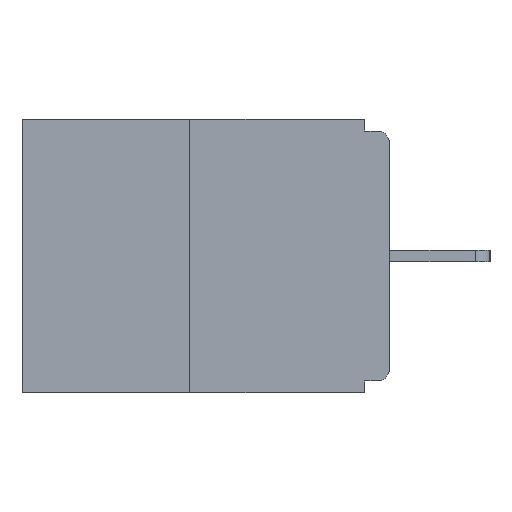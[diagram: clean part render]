
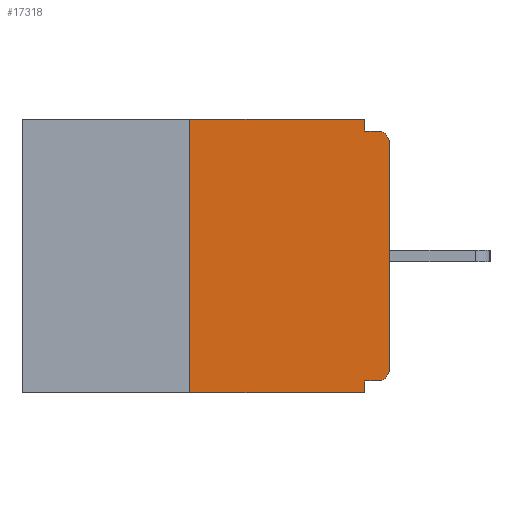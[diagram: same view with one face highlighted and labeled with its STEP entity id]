
A CAD part, left-side view. The second image highlights one B-rep face of the part: STEP entity #17318.
In plain terms, the highlighted planar face has unit normal (-1, 0, 0).
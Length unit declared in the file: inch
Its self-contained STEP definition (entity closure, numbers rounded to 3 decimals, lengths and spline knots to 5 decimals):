
#154 = DIRECTION ( 'NONE',  ( 0., -1., 0. ) ) ;
#231 = DIRECTION ( 'NONE',  ( 0., -1., 0. ) ) ;
#353 = DIRECTION ( 'NONE',  ( 0., 1., 0. ) ) ;
#889 = CARTESIAN_POINT ( 'NONE',  ( 0., 0.031, 0. ) ) ;
#992 = DIRECTION ( 'NONE',  ( 0., 0., -1. ) ) ;
#1017 = VECTOR ( 'NONE', #8878, 39.37008 ) ;
#1216 = VERTEX_POINT ( 'NONE', #3396 ) ;
#1572 = FACE_OUTER_BOUND ( 'NONE', #5780, .T. ) ;
#2127 = VERTEX_POINT ( 'NONE', #9946 ) ;
#2263 = AXIS2_PLACEMENT_3D ( 'NONE', #9028, #4703, #18365 ) ;
#2446 = VERTEX_POINT ( 'NONE', #13920 ) ;
#2466 = CARTESIAN_POINT ( 'NONE',  ( 0., 0.25, 0. ) ) ;
#2790 = LINE ( 'NONE', #10795, #16393 ) ;
#2808 = VECTOR ( 'NONE', #231, 39.37008 ) ;
#3085 = LINE ( 'NONE', #9279, #2808 ) ;
#3396 = CARTESIAN_POINT ( 'NONE',  ( 0., 0.031, -0.343 ) ) ;
#3453 = ORIENTED_EDGE ( 'NONE', *, *, #7222, .F. ) ;
#4030 = EDGE_CURVE ( 'NONE', #13997, #1216, #3085, .T. ) ;
#4128 = ORIENTED_EDGE ( 'NONE', *, *, #18078, .T. ) ;
#4703 = DIRECTION ( 'NONE',  ( -1., 0., 0. ) ) ;
#4943 = CARTESIAN_POINT ( 'NONE',  ( 0., 0., -0.03 ) ) ;
#4972 = LINE ( 'NONE', #18648, #16257 ) ;
#5267 = AXIS2_PLACEMENT_3D ( 'NONE', #12679, #8054, #12485 ) ;
#5558 = VERTEX_POINT ( 'NONE', #19619 ) ;
#5698 = VERTEX_POINT ( 'NONE', #2466 ) ;
#5731 = DIRECTION ( 'NONE',  ( -1., 0., 0. ) ) ;
#5780 = EDGE_LOOP ( 'NONE', ( #3453, #14515, #17949, #17468, #13787, #6718, #7789, #4128, #11120, #6694 ) ) ;
#5939 = DIRECTION ( 'NONE',  ( 0., 0., 1. ) ) ;
#6694 = ORIENTED_EDGE ( 'NONE', *, *, #19433, .F. ) ;
#6718 = ORIENTED_EDGE ( 'NONE', *, *, #12239, .T. ) ;
#6773 = EDGE_CURVE ( 'NONE', #8079, #2127, #4972, .T. ) ;
#6916 = VECTOR ( 'NONE', #17619, 39.37008 ) ;
#6953 = LINE ( 'NONE', #8866, #16837 ) ;
#7222 = EDGE_CURVE ( 'NONE', #5698, #5558, #14438, .T. ) ;
#7484 = VERTEX_POINT ( 'NONE', #16487 ) ;
#7655 = PLANE ( 'NONE',  #5267 ) ;
#7789 = ORIENTED_EDGE ( 'NONE', *, *, #8842, .T. ) ;
#8054 = DIRECTION ( 'NONE',  ( 1., 0., 0. ) ) ;
#8079 = VERTEX_POINT ( 'NONE', #19260 ) ;
#8117 = LINE ( 'NONE', #17078, #18881 ) ;
#8842 = EDGE_CURVE ( 'NONE', #7484, #14604, #8117, .T. ) ;
#8866 = CARTESIAN_POINT ( 'NONE',  ( 0., 0.25, 0. ) ) ;
#8878 = DIRECTION ( 'NONE',  ( 0., 0., -1. ) ) ;
#9028 = CARTESIAN_POINT ( 'NONE',  ( 0., 0.015, -0.313 ) ) ;
#9279 = CARTESIAN_POINT ( 'NONE',  ( 0., 0.46, -0.343 ) ) ;
#9760 = VECTOR ( 'NONE', #992, 39.37008 ) ;
#9946 = CARTESIAN_POINT ( 'NONE',  ( 0., 0.031, -0.328 ) ) ;
#10795 = CARTESIAN_POINT ( 'NONE',  ( 0., 0., -0.015 ) ) ;
#10898 = CARTESIAN_POINT ( 'NONE',  ( 0., 0.25, -0.343 ) ) ;
#11120 = ORIENTED_EDGE ( 'NONE', *, *, #12690, .F. ) ;
#11532 = LINE ( 'NONE', #889, #9760 ) ;
#11969 = CARTESIAN_POINT ( 'NONE',  ( 0., 0.015, -0.03 ) ) ;
#12239 = EDGE_CURVE ( 'NONE', #8079, #7484, #16699, .T. ) ;
#12485 = DIRECTION ( 'NONE',  ( 0., 0., -1. ) ) ;
#12679 = CARTESIAN_POINT ( 'NONE',  ( 0., 0.46, 0. ) ) ;
#12690 = EDGE_CURVE ( 'NONE', #14749, #2446, #2790, .T. ) ;
#13114 = EDGE_CURVE ( 'NONE', #2127, #1216, #13674, .T. ) ;
#13156 = CARTESIAN_POINT ( 'NONE',  ( 0., 0.031, -0.015 ) ) ;
#13212 = CIRCLE ( 'NONE', #19350, 0.015 ) ;
#13674 = LINE ( 'NONE', #18031, #1017 ) ;
#13787 = ORIENTED_EDGE ( 'NONE', *, *, #6773, .F. ) ;
#13920 = CARTESIAN_POINT ( 'NONE',  ( 0., 0.015, -0.015 ) ) ;
#13997 = VERTEX_POINT ( 'NONE', #10898 ) ;
#14438 = LINE ( 'NONE', #14646, #6916 ) ;
#14515 = ORIENTED_EDGE ( 'NONE', *, *, #19787, .F. ) ;
#14604 = VERTEX_POINT ( 'NONE', #4943 ) ;
#14646 = CARTESIAN_POINT ( 'NONE',  ( 0., 0.46, 0. ) ) ;
#14749 = VERTEX_POINT ( 'NONE', #13156 ) ;
#15661 = DIRECTION ( 'NONE',  ( 0., 0., 1. ) ) ;
#16257 = VECTOR ( 'NONE', #353, 39.37008 ) ;
#16393 = VECTOR ( 'NONE', #154, 39.37008 ) ;
#16487 = CARTESIAN_POINT ( 'NONE',  ( 0., 0., -0.313 ) ) ;
#16699 = CIRCLE ( 'NONE', #2263, 0.015 ) ;
#16837 = VECTOR ( 'NONE', #5939, 39.37008 ) ;
#17078 = CARTESIAN_POINT ( 'NONE',  ( 0., 0., 0. ) ) ;
#17318 = ADVANCED_FACE ( 'NONE', ( #1572 ), #7655, .F. ) ;
#17468 = ORIENTED_EDGE ( 'NONE', *, *, #13114, .F. ) ;
#17619 = DIRECTION ( 'NONE',  ( 0., -1., 0. ) ) ;
#17949 = ORIENTED_EDGE ( 'NONE', *, *, #4030, .T. ) ;
#18009 = DIRECTION ( 'NONE',  ( 0., 0., -1. ) ) ;
#18031 = CARTESIAN_POINT ( 'NONE',  ( 0., 0.031, -0.343 ) ) ;
#18078 = EDGE_CURVE ( 'NONE', #14604, #2446, #13212, .T. ) ;
#18365 = DIRECTION ( 'NONE',  ( 0., 0., -1. ) ) ;
#18648 = CARTESIAN_POINT ( 'NONE',  ( 0., 0., -0.328 ) ) ;
#18881 = VECTOR ( 'NONE', #15661, 39.37008 ) ;
#19260 = CARTESIAN_POINT ( 'NONE',  ( 0., 0.015, -0.328 ) ) ;
#19350 = AXIS2_PLACEMENT_3D ( 'NONE', #11969, #5731, #18009 ) ;
#19433 = EDGE_CURVE ( 'NONE', #5558, #14749, #11532, .T. ) ;
#19619 = CARTESIAN_POINT ( 'NONE',  ( 0., 0.031, 0. ) ) ;
#19787 = EDGE_CURVE ( 'NONE', #13997, #5698, #6953, .T. ) ;
